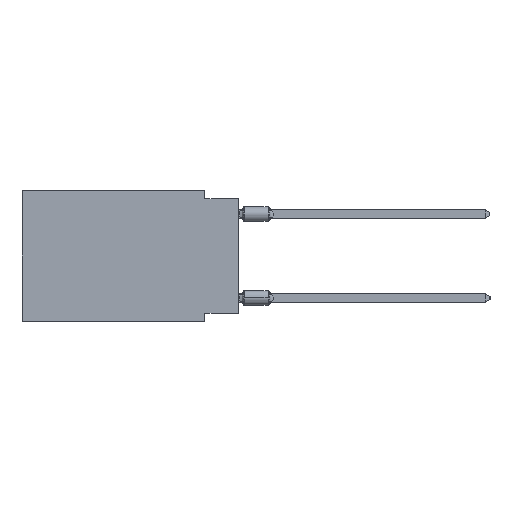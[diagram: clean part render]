
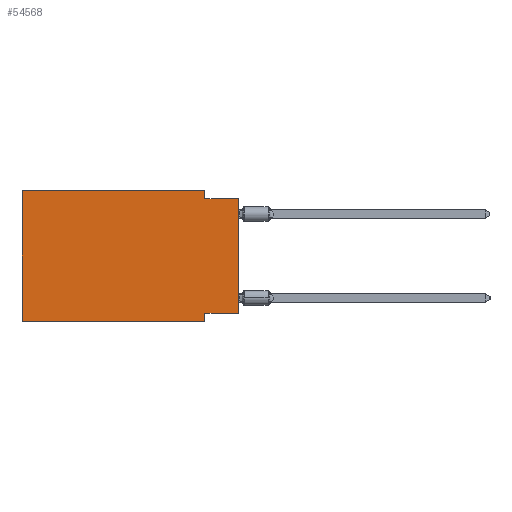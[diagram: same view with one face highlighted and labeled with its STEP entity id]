
A CAD part, left-side view. The second image highlights one B-rep face of the part: STEP entity #54568.
In plain terms, the highlighted planar face has unit normal (-1, 0, 0).
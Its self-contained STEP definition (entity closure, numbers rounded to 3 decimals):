
#638 = VECTOR ( 'NONE', #15320, 1000. ) ;
#1428 = CARTESIAN_POINT ( 'NONE',  ( 0., 16.383, 0. ) ) ;
#3089 = VECTOR ( 'NONE', #51484, 1000. ) ;
#3345 = VERTEX_POINT ( 'NONE', #43862 ) ;
#3671 = VERTEX_POINT ( 'NONE', #21544 ) ;
#8076 = CARTESIAN_POINT ( 'NONE',  ( 0., 2.54, -9.906 ) ) ;
#8440 = EDGE_CURVE ( 'NONE', #28102, #3671, #22188, .T. ) ;
#11055 = LINE ( 'NONE', #36311, #26843 ) ;
#12548 = ORIENTED_EDGE ( 'NONE', *, *, #22194, .F. ) ;
#13520 = CARTESIAN_POINT ( 'NONE',  ( 0., 2.54, 0. ) ) ;
#13952 = DIRECTION ( 'NONE',  ( 0., 0., -1. ) ) ;
#15320 = DIRECTION ( 'NONE',  ( 0., -1., 0. ) ) ;
#15492 = EDGE_LOOP ( 'NONE', ( #45099, #12548, #47782, #45154, #35364, #36731, #43296, #62834 ) ) ;
#17452 = EDGE_CURVE ( 'NONE', #60130, #3345, #11055, .T. ) ;
#17953 = CARTESIAN_POINT ( 'NONE',  ( 0., 2.54, 0. ) ) ;
#18107 = EDGE_CURVE ( 'NONE', #28102, #47583, #31394, .T. ) ;
#20446 = LINE ( 'NONE', #1428, #46839 ) ;
#20863 = CARTESIAN_POINT ( 'NONE',  ( 0., 0., -9.271 ) ) ;
#21544 = CARTESIAN_POINT ( 'NONE',  ( 0., 2.54, -9.271 ) ) ;
#21774 = CARTESIAN_POINT ( 'NONE',  ( 0., 16.383, -9.906 ) ) ;
#22032 = VERTEX_POINT ( 'NONE', #64498 ) ;
#22188 = LINE ( 'NONE', #32360, #37581 ) ;
#22194 = EDGE_CURVE ( 'NONE', #37833, #47583, #51687, .T. ) ;
#22800 = VECTOR ( 'NONE', #57468, 1000. ) ;
#25694 = EDGE_CURVE ( 'NONE', #3345, #56685, #20446, .T. ) ;
#26843 = VECTOR ( 'NONE', #51036, 1000. ) ;
#27405 = CARTESIAN_POINT ( 'NONE',  ( 0., 2.54, -0.635 ) ) ;
#27615 = DIRECTION ( 'NONE',  ( 1., 0., 0. ) ) ;
#27633 = LINE ( 'NONE', #13520, #22800 ) ;
#28070 = LINE ( 'NONE', #8076, #31879 ) ;
#28102 = VERTEX_POINT ( 'NONE', #20863 ) ;
#28256 = DIRECTION ( 'NONE',  ( 0., 0., -1. ) ) ;
#28972 = VECTOR ( 'NONE', #46138, 1000. ) ;
#31394 = LINE ( 'NONE', #55323, #28972 ) ;
#31879 = VECTOR ( 'NONE', #13952, 1000. ) ;
#32360 = CARTESIAN_POINT ( 'NONE',  ( 0., 0., -9.271 ) ) ;
#35364 = ORIENTED_EDGE ( 'NONE', *, *, #17452, .F. ) ;
#35522 = FACE_OUTER_BOUND ( 'NONE', #15492, .T. ) ;
#36311 = CARTESIAN_POINT ( 'NONE',  ( 0., 16.383, 0. ) ) ;
#36731 = ORIENTED_EDGE ( 'NONE', *, *, #37060, .T. ) ;
#37060 = EDGE_CURVE ( 'NONE', #60130, #22032, #58583, .T. ) ;
#37506 = AXIS2_PLACEMENT_3D ( 'NONE', #57765, #27615, #28256 ) ;
#37581 = VECTOR ( 'NONE', #52354, 1000. ) ;
#37833 = VERTEX_POINT ( 'NONE', #27405 ) ;
#42622 = CARTESIAN_POINT ( 'NONE',  ( 0., 0., -0.635 ) ) ;
#43296 = ORIENTED_EDGE ( 'NONE', *, *, #59808, .F. ) ;
#43862 = CARTESIAN_POINT ( 'NONE',  ( 0., 16.383, 0. ) ) ;
#45099 = ORIENTED_EDGE ( 'NONE', *, *, #18107, .T. ) ;
#45154 = ORIENTED_EDGE ( 'NONE', *, *, #25694, .F. ) ;
#45698 = DIRECTION ( 'NONE',  ( 0., -1., 0. ) ) ;
#46138 = DIRECTION ( 'NONE',  ( 0., 0., 1. ) ) ;
#46588 = CARTESIAN_POINT ( 'NONE',  ( 0., 16.383, -9.906 ) ) ;
#46839 = VECTOR ( 'NONE', #45698, 1000. ) ;
#47583 = VERTEX_POINT ( 'NONE', #42622 ) ;
#47782 = ORIENTED_EDGE ( 'NONE', *, *, #52152, .F. ) ;
#50589 = PLANE ( 'NONE',  #37506 ) ;
#51036 = DIRECTION ( 'NONE',  ( 0., 0., 1. ) ) ;
#51484 = DIRECTION ( 'NONE',  ( 0., -1., 0. ) ) ;
#51687 = LINE ( 'NONE', #60560, #638 ) ;
#52152 = EDGE_CURVE ( 'NONE', #56685, #37833, #27633, .T. ) ;
#52354 = DIRECTION ( 'NONE',  ( 0., 1., 0. ) ) ;
#54568 = ADVANCED_FACE ( 'NONE', ( #35522 ), #50589, .F. ) ;
#55323 = CARTESIAN_POINT ( 'NONE',  ( 0., 0., 0. ) ) ;
#56685 = VERTEX_POINT ( 'NONE', #17953 ) ;
#57468 = DIRECTION ( 'NONE',  ( 0., 0., -1. ) ) ;
#57765 = CARTESIAN_POINT ( 'NONE',  ( 0., 16.383, 0. ) ) ;
#58583 = LINE ( 'NONE', #46588, #3089 ) ;
#59808 = EDGE_CURVE ( 'NONE', #3671, #22032, #28070, .T. ) ;
#60130 = VERTEX_POINT ( 'NONE', #21774 ) ;
#60560 = CARTESIAN_POINT ( 'NONE',  ( 0., 0., -0.635 ) ) ;
#62834 = ORIENTED_EDGE ( 'NONE', *, *, #8440, .F. ) ;
#64498 = CARTESIAN_POINT ( 'NONE',  ( 0., 2.54, -9.906 ) ) ;
